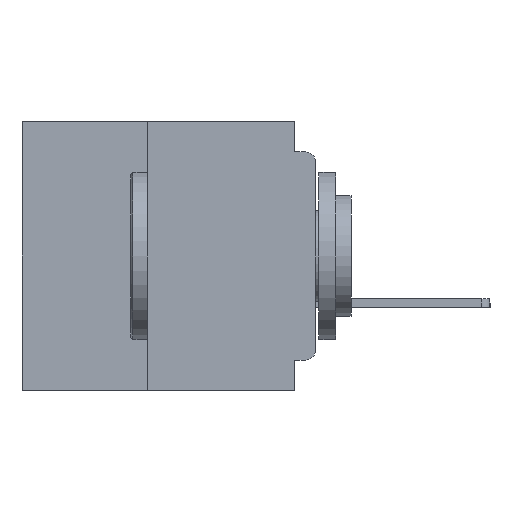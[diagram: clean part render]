
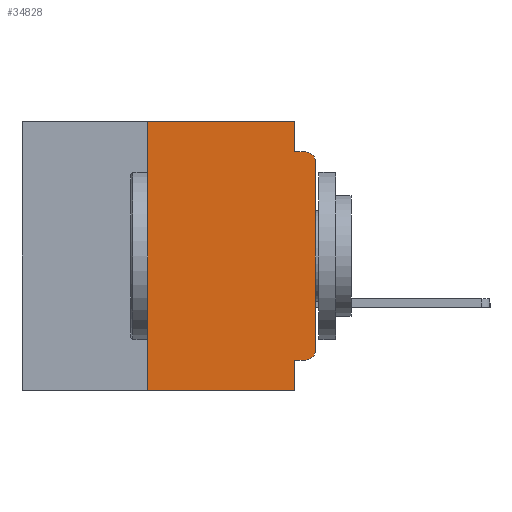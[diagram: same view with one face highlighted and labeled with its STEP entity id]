
A CAD part, left-side view. The second image highlights one B-rep face of the part: STEP entity #34828.
In plain terms, the highlighted planar face has unit normal (-1, 0, 0).
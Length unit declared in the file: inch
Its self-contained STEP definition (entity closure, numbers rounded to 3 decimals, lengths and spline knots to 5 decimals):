
#1757 = LINE ( 'NONE', #18252, #39944 ) ;
#2263 = EDGE_CURVE ( 'NONE', #13918, #26769, #40207, .T. ) ;
#2604 = VECTOR ( 'NONE', #10829, 39.37008 ) ;
#2616 = LINE ( 'NONE', #16872, #26891 ) ;
#2946 = EDGE_CURVE ( 'NONE', #27048, #12585, #37657, .T. ) ;
#3607 = DIRECTION ( 'NONE',  ( 0., -1., 0. ) ) ;
#4199 = CARTESIAN_POINT ( 'NONE',  ( 0., 0.015, -0.355 ) ) ;
#4306 = CARTESIAN_POINT ( 'NONE',  ( 0., 0.25, 0. ) ) ;
#4348 = VERTEX_POINT ( 'NONE', #4306 ) ;
#4432 = CARTESIAN_POINT ( 'NONE',  ( 0., 0.437, -0.4 ) ) ;
#4878 = CARTESIAN_POINT ( 'NONE',  ( 0., 0.015, -0.06 ) ) ;
#5069 = EDGE_LOOP ( 'NONE', ( #16169, #18120, #35557, #35048, #13745, #19601, #12533, #26262, #6691, #15272 ) ) ;
#5890 = CARTESIAN_POINT ( 'NONE',  ( 0., 0., 0. ) ) ;
#5915 = CARTESIAN_POINT ( 'NONE',  ( 0., 0.015, -0.34 ) ) ;
#5962 = DIRECTION ( 'NONE',  ( -1., 0., 0. ) ) ;
#6179 = VECTOR ( 'NONE', #15476, 39.37008 ) ;
#6476 = EDGE_CURVE ( 'NONE', #11142, #12585, #28877, .T. ) ;
#6571 = VECTOR ( 'NONE', #35111, 39.37008 ) ;
#6572 = CARTESIAN_POINT ( 'NONE',  ( 0., 0., -0.355 ) ) ;
#6691 = ORIENTED_EDGE ( 'NONE', *, *, #13773, .F. ) ;
#7290 = CIRCLE ( 'NONE', #21851, 0.015 ) ;
#8070 = DIRECTION ( 'NONE',  ( 0., 0., -1. ) ) ;
#10829 = DIRECTION ( 'NONE',  ( 0., 0., -1. ) ) ;
#11011 = CARTESIAN_POINT ( 'NONE',  ( 0., 0.031, -0.4 ) ) ;
#11056 = AXIS2_PLACEMENT_3D ( 'NONE', #5915, #5962, #26780 ) ;
#11142 = VERTEX_POINT ( 'NONE', #27450 ) ;
#11672 = AXIS2_PLACEMENT_3D ( 'NONE', #34514, #37677, #18679 ) ;
#11845 = EDGE_CURVE ( 'NONE', #4348, #32244, #1757, .T. ) ;
#11868 = CARTESIAN_POINT ( 'NONE',  ( 0., 0.031, -0.045 ) ) ;
#12016 = DIRECTION ( 'NONE',  ( 0., -1., 0. ) ) ;
#12278 = CARTESIAN_POINT ( 'NONE',  ( 0., 0.25, -0.4 ) ) ;
#12296 = PLANE ( 'NONE',  #11672 ) ;
#12316 = CARTESIAN_POINT ( 'NONE',  ( 0., 0.25, -0.4 ) ) ;
#12345 = VECTOR ( 'NONE', #3607, 39.37008 ) ;
#12533 = ORIENTED_EDGE ( 'NONE', *, *, #2946, .T. ) ;
#12585 = VERTEX_POINT ( 'NONE', #28042 ) ;
#13640 = EDGE_CURVE ( 'NONE', #26769, #20637, #28369, .T. ) ;
#13745 = ORIENTED_EDGE ( 'NONE', *, *, #11845, .F. ) ;
#13773 = EDGE_CURVE ( 'NONE', #13918, #11142, #14958, .T. ) ;
#13918 = VERTEX_POINT ( 'NONE', #4199 ) ;
#14684 = VERTEX_POINT ( 'NONE', #11868 ) ;
#14958 = LINE ( 'NONE', #6572, #6571 ) ;
#15258 = EDGE_CURVE ( 'NONE', #14684, #20277, #18307, .T. ) ;
#15272 = ORIENTED_EDGE ( 'NONE', *, *, #2263, .T. ) ;
#15476 = DIRECTION ( 'NONE',  ( 0., 0., 1. ) ) ;
#16169 = ORIENTED_EDGE ( 'NONE', *, *, #13640, .T. ) ;
#16872 = CARTESIAN_POINT ( 'NONE',  ( 0., 0.031, 0. ) ) ;
#17063 = EDGE_CURVE ( 'NONE', #32244, #14684, #2616, .T. ) ;
#18120 = ORIENTED_EDGE ( 'NONE', *, *, #36617, .T. ) ;
#18252 = CARTESIAN_POINT ( 'NONE',  ( 0., 0.437, 0. ) ) ;
#18307 = LINE ( 'NONE', #39983, #33212 ) ;
#18679 = DIRECTION ( 'NONE',  ( 0., 0., -1. ) ) ;
#19601 = ORIENTED_EDGE ( 'NONE', *, *, #26176, .F. ) ;
#20277 = VERTEX_POINT ( 'NONE', #24495 ) ;
#20637 = VERTEX_POINT ( 'NONE', #32817 ) ;
#20711 = DIRECTION ( 'NONE',  ( 0., -1., 0. ) ) ;
#21538 = CARTESIAN_POINT ( 'NONE',  ( 0., 0., -0.34 ) ) ;
#21851 = AXIS2_PLACEMENT_3D ( 'NONE', #4878, #27027, #8070 ) ;
#23255 = DIRECTION ( 'NONE',  ( 0., 0., -1. ) ) ;
#24495 = CARTESIAN_POINT ( 'NONE',  ( 0., 0.015, -0.045 ) ) ;
#26176 = EDGE_CURVE ( 'NONE', #27048, #4348, #31471, .T. ) ;
#26262 = ORIENTED_EDGE ( 'NONE', *, *, #6476, .F. ) ;
#26769 = VERTEX_POINT ( 'NONE', #21538 ) ;
#26780 = DIRECTION ( 'NONE',  ( 0., 0., -1. ) ) ;
#26891 = VECTOR ( 'NONE', #23255, 39.37008 ) ;
#27027 = DIRECTION ( 'NONE',  ( -1., 0., 0. ) ) ;
#27048 = VERTEX_POINT ( 'NONE', #12316 ) ;
#27450 = CARTESIAN_POINT ( 'NONE',  ( 0., 0.031, -0.355 ) ) ;
#28028 = DIRECTION ( 'NONE',  ( 0., 0., 1. ) ) ;
#28042 = CARTESIAN_POINT ( 'NONE',  ( 0., 0.031, -0.4 ) ) ;
#28369 = LINE ( 'NONE', #5890, #35817 ) ;
#28877 = LINE ( 'NONE', #11011, #2604 ) ;
#31471 = LINE ( 'NONE', #12278, #6179 ) ;
#32244 = VERTEX_POINT ( 'NONE', #33442 ) ;
#32817 = CARTESIAN_POINT ( 'NONE',  ( 0., 0., -0.06 ) ) ;
#33212 = VECTOR ( 'NONE', #20711, 39.37008 ) ;
#33442 = CARTESIAN_POINT ( 'NONE',  ( 0., 0.031, 0. ) ) ;
#34514 = CARTESIAN_POINT ( 'NONE',  ( 0., 0.437, 0. ) ) ;
#34828 = ADVANCED_FACE ( 'NONE', ( #35715 ), #12296, .F. ) ;
#35048 = ORIENTED_EDGE ( 'NONE', *, *, #17063, .F. ) ;
#35111 = DIRECTION ( 'NONE',  ( 0., 1., 0. ) ) ;
#35557 = ORIENTED_EDGE ( 'NONE', *, *, #15258, .F. ) ;
#35715 = FACE_OUTER_BOUND ( 'NONE', #5069, .T. ) ;
#35817 = VECTOR ( 'NONE', #28028, 39.37008 ) ;
#36617 = EDGE_CURVE ( 'NONE', #20637, #20277, #7290, .T. ) ;
#37657 = LINE ( 'NONE', #4432, #12345 ) ;
#37677 = DIRECTION ( 'NONE',  ( 1., 0., 0. ) ) ;
#39944 = VECTOR ( 'NONE', #12016, 39.37008 ) ;
#39983 = CARTESIAN_POINT ( 'NONE',  ( 0., 0., -0.045 ) ) ;
#40207 = CIRCLE ( 'NONE', #11056, 0.015 ) ;
